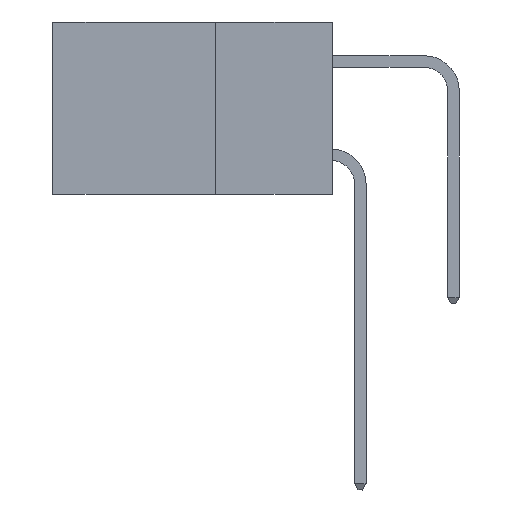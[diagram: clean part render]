
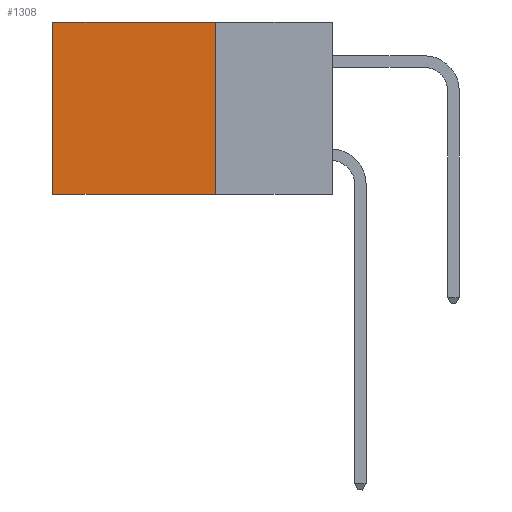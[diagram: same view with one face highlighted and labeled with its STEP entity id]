
A CAD part, left-side view. The second image highlights one B-rep face of the part: STEP entity #1308.
In plain terms, the highlighted planar face has unit normal (-1, 0, 0).
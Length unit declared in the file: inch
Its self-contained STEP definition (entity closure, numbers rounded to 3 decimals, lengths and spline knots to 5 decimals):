
#1058 = CARTESIAN_POINT ( 'NONE',  ( 0.298, 0.25, 0. ) ) ;
#1308 = ADVANCED_FACE ( 'NONE', ( #2947 ), #2340, .F. ) ;
#1559 = LINE ( 'NONE', #7290, #5980 ) ;
#2302 = EDGE_CURVE ( 'NONE', #14426, #6609, #6960, .T. ) ;
#2340 = PLANE ( 'NONE',  #13761 ) ;
#2914 = CARTESIAN_POINT ( 'NONE',  ( 0.298, 0.25, -0.37 ) ) ;
#2947 = FACE_OUTER_BOUND ( 'NONE', #9291, .T. ) ;
#3825 = DIRECTION ( 'NONE',  ( 0., 1., 0. ) ) ;
#4134 = ORIENTED_EDGE ( 'NONE', *, *, #8263, .T. ) ;
#4305 = ORIENTED_EDGE ( 'NONE', *, *, #11666, .F. ) ;
#4857 = EDGE_CURVE ( 'NONE', #8655, #16611, #7476, .T. ) ;
#4891 = DIRECTION ( 'NONE',  ( 0., 0., -1. ) ) ;
#5111 = VECTOR ( 'NONE', #11792, 39.37008 ) ;
#5588 = ORIENTED_EDGE ( 'NONE', *, *, #4857, .F. ) ;
#5776 = DIRECTION ( 'NONE',  ( 0., 1., 0. ) ) ;
#5980 = VECTOR ( 'NONE', #3825, 39.37008 ) ;
#6609 = VERTEX_POINT ( 'NONE', #8851 ) ;
#6960 = LINE ( 'NONE', #9086, #5111 ) ;
#7030 = CARTESIAN_POINT ( 'NONE',  ( 0.298, 0.25, 0. ) ) ;
#7290 = CARTESIAN_POINT ( 'NONE',  ( 0.298, 0.25, -0.37 ) ) ;
#7428 = DIRECTION ( 'NONE',  ( 0., 0., -1. ) ) ;
#7476 = LINE ( 'NONE', #12604, #16208 ) ;
#7539 = DIRECTION ( 'NONE',  ( 1., 0., 0. ) ) ;
#8263 = EDGE_CURVE ( 'NONE', #8655, #14426, #8969, .T. ) ;
#8655 = VERTEX_POINT ( 'NONE', #1058 ) ;
#8851 = CARTESIAN_POINT ( 'NONE',  ( 0.298, 0.6, -0.37 ) ) ;
#8969 = LINE ( 'NONE', #7030, #14679 ) ;
#9086 = CARTESIAN_POINT ( 'NONE',  ( 0.298, 0.6, 0. ) ) ;
#9291 = EDGE_LOOP ( 'NONE', ( #14594, #4305, #5588, #4134 ) ) ;
#11666 = EDGE_CURVE ( 'NONE', #16611, #6609, #1559, .T. ) ;
#11792 = DIRECTION ( 'NONE',  ( 0., 0., -1. ) ) ;
#12575 = CARTESIAN_POINT ( 'NONE',  ( 0.298, 0.25, 0. ) ) ;
#12604 = CARTESIAN_POINT ( 'NONE',  ( 0.298, 0.25, 0. ) ) ;
#12972 = CARTESIAN_POINT ( 'NONE',  ( 0.298, 0.6, 0. ) ) ;
#13761 = AXIS2_PLACEMENT_3D ( 'NONE', #12575, #7539, #7428 ) ;
#14426 = VERTEX_POINT ( 'NONE', #12972 ) ;
#14594 = ORIENTED_EDGE ( 'NONE', *, *, #2302, .T. ) ;
#14679 = VECTOR ( 'NONE', #5776, 39.37008 ) ;
#16208 = VECTOR ( 'NONE', #4891, 39.37008 ) ;
#16611 = VERTEX_POINT ( 'NONE', #2914 ) ;
